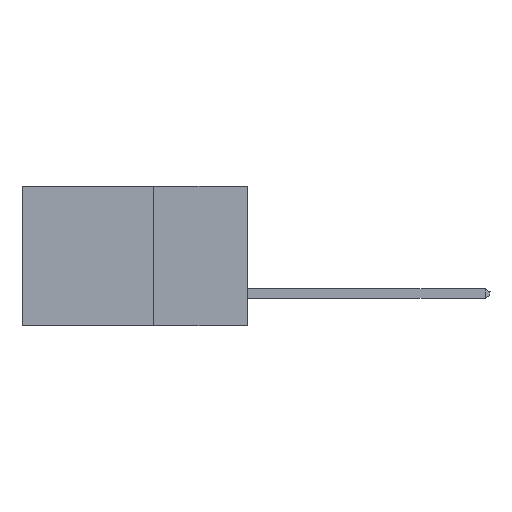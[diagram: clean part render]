
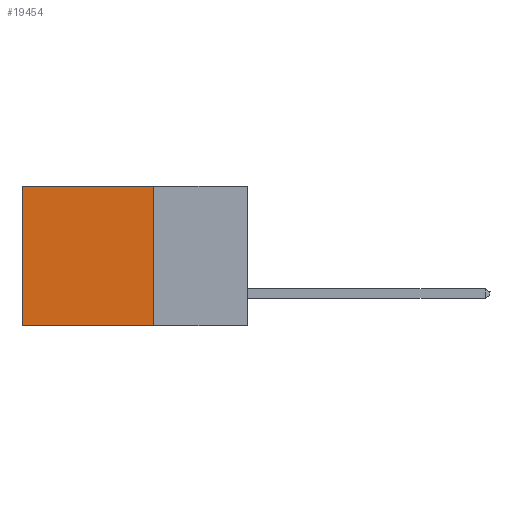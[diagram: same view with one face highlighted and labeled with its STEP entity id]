
A CAD part, left-side view. The second image highlights one B-rep face of the part: STEP entity #19454.
In plain terms, the highlighted planar face has unit normal (-1, 0, 0).
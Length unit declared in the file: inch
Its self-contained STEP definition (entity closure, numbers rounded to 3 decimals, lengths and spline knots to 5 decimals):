
#859 = EDGE_CURVE ( 'NONE', #4608, #9908, #9454, .T. ) ;
#1410 = AXIS2_PLACEMENT_3D ( 'NONE', #10748, #18414, #10876 ) ;
#1851 = DIRECTION ( 'NONE',  ( 0., 0., -1. ) ) ;
#1876 = CARTESIAN_POINT ( 'NONE',  ( 0.2615, 0.6, -0.37 ) ) ;
#3288 = VERTEX_POINT ( 'NONE', #22745 ) ;
#3400 = CARTESIAN_POINT ( 'NONE',  ( 0.2615, 0.6, -0.37 ) ) ;
#3625 = FACE_OUTER_BOUND ( 'NONE', #22741, .T. ) ;
#4608 = VERTEX_POINT ( 'NONE', #16700 ) ;
#6795 = CARTESIAN_POINT ( 'NONE',  ( 0.2615, 0.25, 0. ) ) ;
#7655 = CARTESIAN_POINT ( 'NONE',  ( 0.2615, 0.25, 0. ) ) ;
#8608 = ORIENTED_EDGE ( 'NONE', *, *, #859, .F. ) ;
#9454 = LINE ( 'NONE', #14974, #13847 ) ;
#9740 = VECTOR ( 'NONE', #15289, 39.37008 ) ;
#9796 = EDGE_CURVE ( 'NONE', #3288, #9908, #14804, .T. ) ;
#9908 = VERTEX_POINT ( 'NONE', #3400 ) ;
#10693 = ORIENTED_EDGE ( 'NONE', *, *, #9796, .T. ) ;
#10748 = CARTESIAN_POINT ( 'NONE',  ( 0.2615, 0.25, -0.37 ) ) ;
#10876 = DIRECTION ( 'NONE',  ( 0., 0., -1. ) ) ;
#11164 = ORIENTED_EDGE ( 'NONE', *, *, #19600, .F. ) ;
#11365 = LINE ( 'NONE', #19012, #16629 ) ;
#13847 = VECTOR ( 'NONE', #18610, 39.37008 ) ;
#14529 = PLANE ( 'NONE',  #1410 ) ;
#14804 = LINE ( 'NONE', #1876, #18026 ) ;
#14974 = CARTESIAN_POINT ( 'NONE',  ( 0.2615, 0.25, -0.37 ) ) ;
#15285 = DIRECTION ( 'NONE',  ( 0., 0., -1. ) ) ;
#15289 = DIRECTION ( 'NONE',  ( 0., 1., 0. ) ) ;
#15501 = VERTEX_POINT ( 'NONE', #6795 ) ;
#15771 = EDGE_CURVE ( 'NONE', #15501, #3288, #17675, .T. ) ;
#16629 = VECTOR ( 'NONE', #1851, 39.37008 ) ;
#16700 = CARTESIAN_POINT ( 'NONE',  ( 0.2615, 0.25, -0.37 ) ) ;
#17675 = LINE ( 'NONE', #7655, #9740 ) ;
#18026 = VECTOR ( 'NONE', #15285, 39.37008 ) ;
#18414 = DIRECTION ( 'NONE',  ( 1., 0., 0. ) ) ;
#18610 = DIRECTION ( 'NONE',  ( 0., 1., 0. ) ) ;
#19012 = CARTESIAN_POINT ( 'NONE',  ( 0.2615, 0.25, -0.37 ) ) ;
#19454 = ADVANCED_FACE ( 'NONE', ( #3625 ), #14529, .F. ) ;
#19600 = EDGE_CURVE ( 'NONE', #15501, #4608, #11365, .T. ) ;
#22741 = EDGE_LOOP ( 'NONE', ( #10693, #8608, #11164, #23176 ) ) ;
#22745 = CARTESIAN_POINT ( 'NONE',  ( 0.2615, 0.6, 0. ) ) ;
#23176 = ORIENTED_EDGE ( 'NONE', *, *, #15771, .T. ) ;
